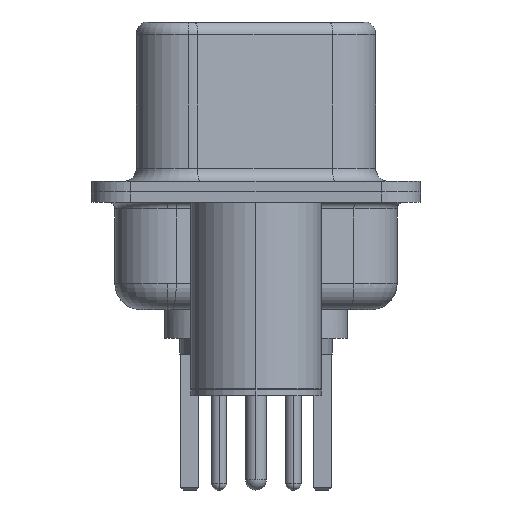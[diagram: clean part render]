
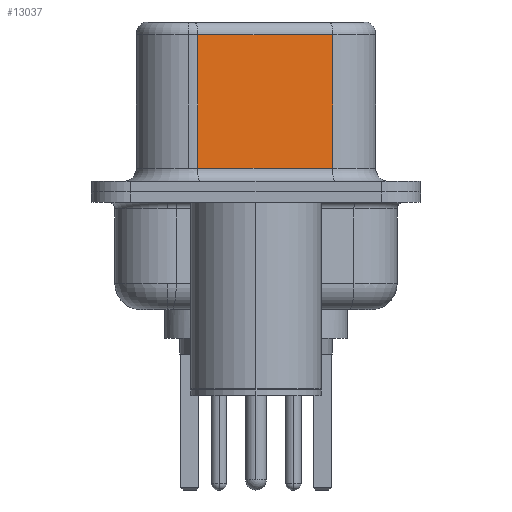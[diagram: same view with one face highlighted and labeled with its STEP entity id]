
A CAD part, left-side view. The second image highlights one B-rep face of the part: STEP entity #13037.
In plain terms, the highlighted planar face has unit normal (-0.985, -0.174, 0).
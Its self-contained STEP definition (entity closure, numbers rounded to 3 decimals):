
#109 = LINE ( 'NONE', #2507, #9587 ) ;
#328 = VECTOR ( 'NONE', #1518, 1000. ) ;
#1501 = ORIENTED_EDGE ( 'NONE', *, *, #5914, .T. ) ;
#1512 = LINE ( 'NONE', #7072, #328 ) ;
#1518 = DIRECTION ( 'NONE',  ( 0., 0., -1. ) ) ;
#2507 = CARTESIAN_POINT ( 'NONE',  ( 4.585, -2.927, 0.9 ) ) ;
#2716 = CARTESIAN_POINT ( 'NONE',  ( 3.675, 2.233, 0.9 ) ) ;
#3926 = VERTEX_POINT ( 'NONE', #6678 ) ;
#4159 = ORIENTED_EDGE ( 'NONE', *, *, #12844, .T. ) ;
#4667 = EDGE_LOOP ( 'NONE', ( #21960, #6998, #1501, #4159 ) ) ;
#5135 = DIRECTION ( 'NONE',  ( 0.985, 0.174, 0. ) ) ;
#5881 = VECTOR ( 'NONE', #13080, 1000. ) ;
#5914 = EDGE_CURVE ( 'NONE', #3926, #18006, #1512, .T. ) ;
#6678 = CARTESIAN_POINT ( 'NONE',  ( 3.675, 2.233, 6.02 ) ) ;
#6998 = ORIENTED_EDGE ( 'NONE', *, *, #21429, .T. ) ;
#7036 = VERTEX_POINT ( 'NONE', #9940 ) ;
#7072 = CARTESIAN_POINT ( 'NONE',  ( 3.675, 2.233, 6.52 ) ) ;
#8688 = CARTESIAN_POINT ( 'NONE',  ( 4.585, -2.927, 6.02 ) ) ;
#9290 = VECTOR ( 'NONE', #21505, 1000. ) ;
#9587 = VECTOR ( 'NONE', #15579, 1000. ) ;
#9940 = CARTESIAN_POINT ( 'NONE',  ( 4.585, -2.927, 0.9 ) ) ;
#10067 = AXIS2_PLACEMENT_3D ( 'NONE', #23464, #5135, #18056 ) ;
#10908 = LINE ( 'NONE', #16646, #5881 ) ;
#12844 = EDGE_CURVE ( 'NONE', #18006, #7036, #109, .T. ) ;
#13037 = ADVANCED_FACE ( 'NONE', ( #20719 ), #19783, .F. ) ;
#13080 = DIRECTION ( 'NONE',  ( 0., 0., -1. ) ) ;
#15579 = DIRECTION ( 'NONE',  ( 0.174, -0.985, 0. ) ) ;
#16646 = CARTESIAN_POINT ( 'NONE',  ( 4.585, -2.927, 6.52 ) ) ;
#17701 = CARTESIAN_POINT ( 'NONE',  ( 4.585, -2.927, 6.02 ) ) ;
#17704 = EDGE_CURVE ( 'NONE', #21369, #7036, #10908, .T. ) ;
#18006 = VERTEX_POINT ( 'NONE', #2716 ) ;
#18056 = DIRECTION ( 'NONE',  ( -0.174, 0.985, 0. ) ) ;
#19783 = PLANE ( 'NONE',  #10067 ) ;
#20139 = LINE ( 'NONE', #8688, #9290 ) ;
#20719 = FACE_OUTER_BOUND ( 'NONE', #4667, .T. ) ;
#21369 = VERTEX_POINT ( 'NONE', #17701 ) ;
#21429 = EDGE_CURVE ( 'NONE', #21369, #3926, #20139, .T. ) ;
#21505 = DIRECTION ( 'NONE',  ( -0.174, 0.985, 0. ) ) ;
#21960 = ORIENTED_EDGE ( 'NONE', *, *, #17704, .F. ) ;
#23464 = CARTESIAN_POINT ( 'NONE',  ( 4.585, -2.927, 6.52 ) ) ;
